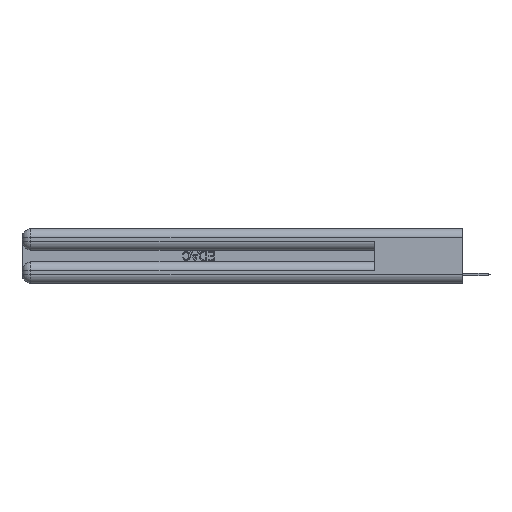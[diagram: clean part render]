
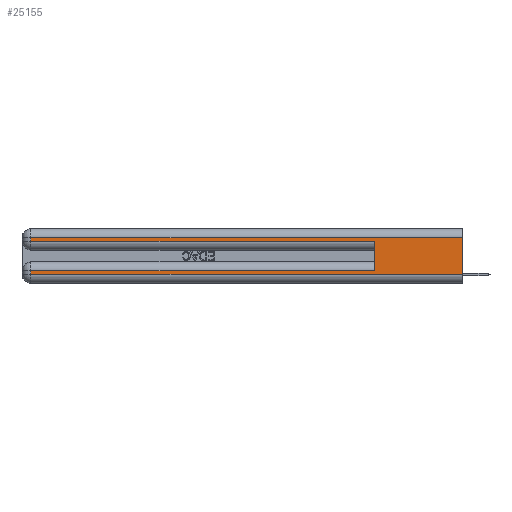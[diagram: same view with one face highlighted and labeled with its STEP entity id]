
A CAD part, left-side view. The second image highlights one B-rep face of the part: STEP entity #25155.
In plain terms, the highlighted planar face has unit normal (-1, 0, 0).
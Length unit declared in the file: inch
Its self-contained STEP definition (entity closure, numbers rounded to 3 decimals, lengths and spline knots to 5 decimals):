
#498 = ORIENTED_EDGE ( 'NONE', *, *, #4480, .T. ) ;
#1501 = CARTESIAN_POINT ( 'NONE',  ( 0., 2.94, 0.31 ) ) ;
#1543 = VECTOR ( 'NONE', #29298, 39.37008 ) ;
#2236 = VERTEX_POINT ( 'NONE', #1501 ) ;
#2694 = VECTOR ( 'NONE', #30017, 39.37008 ) ;
#4480 = EDGE_CURVE ( 'NONE', #18342, #7124, #23788, .T. ) ;
#4527 = VECTOR ( 'NONE', #15077, 39.37008 ) ;
#4805 = ORIENTED_EDGE ( 'NONE', *, *, #22621, .F. ) ;
#5013 = CARTESIAN_POINT ( 'NONE',  ( 0., 0., 0.31 ) ) ;
#5171 = VECTOR ( 'NONE', #18706, 39.37008 ) ;
#5582 = LINE ( 'NONE', #32075, #5171 ) ;
#5629 = EDGE_CURVE ( 'NONE', #7779, #24911, #20757, .T. ) ;
#7124 = VERTEX_POINT ( 'NONE', #33230 ) ;
#7293 = DIRECTION ( 'NONE',  ( 0., 0., -1. ) ) ;
#7517 = CARTESIAN_POINT ( 'NONE',  ( 0., 0., 0.37 ) ) ;
#7602 = DIRECTION ( 'NONE',  ( 0., 1., 0. ) ) ;
#7779 = VERTEX_POINT ( 'NONE', #25930 ) ;
#8279 = CARTESIAN_POINT ( 'NONE',  ( 0., 0., 0.31 ) ) ;
#9519 = CARTESIAN_POINT ( 'NONE',  ( 0., 0., 0.37 ) ) ;
#10539 = VERTEX_POINT ( 'NONE', #8279 ) ;
#10838 = ORIENTED_EDGE ( 'NONE', *, *, #15777, .F. ) ;
#10949 = CARTESIAN_POINT ( 'NONE',  ( 0., 0., 0.085 ) ) ;
#10968 = LINE ( 'NONE', #27632, #14746 ) ;
#11005 = LINE ( 'NONE', #25744, #24467 ) ;
#11675 = ORIENTED_EDGE ( 'NONE', *, *, #28790, .T. ) ;
#12517 = CARTESIAN_POINT ( 'NONE',  ( 0., 0.6, 0.285 ) ) ;
#12525 = EDGE_CURVE ( 'NONE', #2236, #31093, #10968, .T. ) ;
#13778 = CARTESIAN_POINT ( 'NONE',  ( 0., 0., 0.06 ) ) ;
#14520 = CARTESIAN_POINT ( 'NONE',  ( 0., 2.94, 0.285 ) ) ;
#14746 = VECTOR ( 'NONE', #25070, 39.37008 ) ;
#15077 = DIRECTION ( 'NONE',  ( 0., -1., 0. ) ) ;
#15141 = ORIENTED_EDGE ( 'NONE', *, *, #31451, .T. ) ;
#15777 = EDGE_CURVE ( 'NONE', #10539, #24911, #17899, .T. ) ;
#17615 = PLANE ( 'NONE',  #26649 ) ;
#17882 = LINE ( 'NONE', #5013, #22517 ) ;
#17899 = LINE ( 'NONE', #7517, #20816 ) ;
#18342 = VERTEX_POINT ( 'NONE', #18756 ) ;
#18706 = DIRECTION ( 'NONE',  ( 0., 0., 1. ) ) ;
#18756 = CARTESIAN_POINT ( 'NONE',  ( 0., 0.6, 0.085 ) ) ;
#18873 = FACE_OUTER_BOUND ( 'NONE', #21485, .T. ) ;
#19230 = EDGE_CURVE ( 'NONE', #31093, #30681, #25970, .T. ) ;
#20757 = LINE ( 'NONE', #13778, #2694 ) ;
#20816 = VECTOR ( 'NONE', #7293, 39.37008 ) ;
#21485 = EDGE_LOOP ( 'NONE', ( #10838, #11675, #28524, #33460, #4805, #498, #15141, #26579 ) ) ;
#22517 = VECTOR ( 'NONE', #7602, 39.37008 ) ;
#22621 = EDGE_CURVE ( 'NONE', #18342, #30681, #5582, .T. ) ;
#23788 = LINE ( 'NONE', #10949, #1543 ) ;
#24467 = VECTOR ( 'NONE', #28553, 39.37008 ) ;
#24911 = VERTEX_POINT ( 'NONE', #27151 ) ;
#25070 = DIRECTION ( 'NONE',  ( 0., 0., -1. ) ) ;
#25155 = ADVANCED_FACE ( 'NONE', ( #18873 ), #17615, .F. ) ;
#25744 = CARTESIAN_POINT ( 'NONE',  ( 0., 2.94, 0.37 ) ) ;
#25930 = CARTESIAN_POINT ( 'NONE',  ( 0., 2.94, 0.06 ) ) ;
#25970 = LINE ( 'NONE', #33644, #4527 ) ;
#26579 = ORIENTED_EDGE ( 'NONE', *, *, #5629, .T. ) ;
#26649 = AXIS2_PLACEMENT_3D ( 'NONE', #9519, #28643, #31015 ) ;
#27151 = CARTESIAN_POINT ( 'NONE',  ( 0., 0., 0.06 ) ) ;
#27632 = CARTESIAN_POINT ( 'NONE',  ( 0., 2.94, 0.37 ) ) ;
#28524 = ORIENTED_EDGE ( 'NONE', *, *, #12525, .T. ) ;
#28553 = DIRECTION ( 'NONE',  ( 0., 0., -1. ) ) ;
#28643 = DIRECTION ( 'NONE',  ( 1., 0., 0. ) ) ;
#28790 = EDGE_CURVE ( 'NONE', #10539, #2236, #17882, .T. ) ;
#29298 = DIRECTION ( 'NONE',  ( 0., 1., 0. ) ) ;
#30017 = DIRECTION ( 'NONE',  ( 0., -1., 0. ) ) ;
#30681 = VERTEX_POINT ( 'NONE', #12517 ) ;
#31015 = DIRECTION ( 'NONE',  ( 0., 0., -1. ) ) ;
#31093 = VERTEX_POINT ( 'NONE', #14520 ) ;
#31451 = EDGE_CURVE ( 'NONE', #7124, #7779, #11005, .T. ) ;
#32075 = CARTESIAN_POINT ( 'NONE',  ( 0., 0.6, 0.145 ) ) ;
#33230 = CARTESIAN_POINT ( 'NONE',  ( 0., 2.94, 0.085 ) ) ;
#33460 = ORIENTED_EDGE ( 'NONE', *, *, #19230, .T. ) ;
#33644 = CARTESIAN_POINT ( 'NONE',  ( 0., 0., 0.285 ) ) ;
